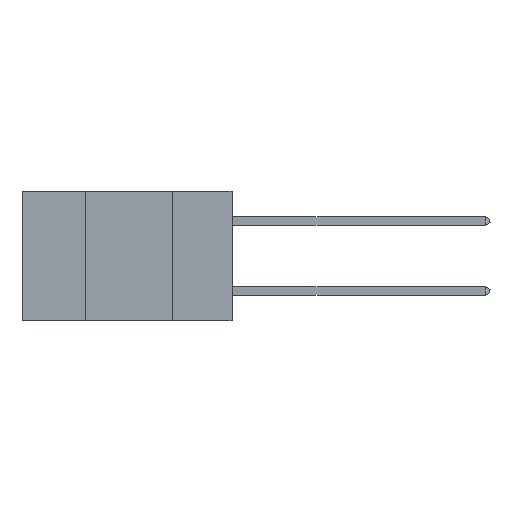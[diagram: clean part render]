
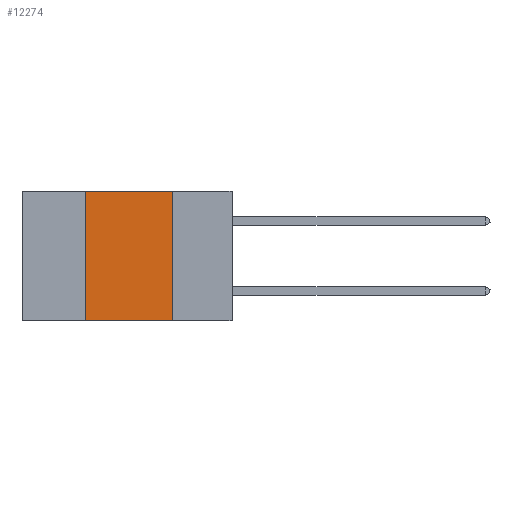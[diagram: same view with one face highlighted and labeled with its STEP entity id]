
A CAD part, left-side view. The second image highlights one B-rep face of the part: STEP entity #12274.
In plain terms, the highlighted planar face has unit normal (-1, 0, 0).
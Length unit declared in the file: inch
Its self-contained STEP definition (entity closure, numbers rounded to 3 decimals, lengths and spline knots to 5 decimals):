
#4 = EDGE_CURVE ( 'NONE', #7648, #14621, #4949, .T. ) ;
#509 = EDGE_CURVE ( 'NONE', #6425, #7648, #12445, .T. ) ;
#868 = DIRECTION ( 'NONE',  ( 0., -1., 0. ) ) ;
#1037 = EDGE_LOOP ( 'NONE', ( #7415, #4270, #7831, #11387 ) ) ;
#1238 = VECTOR ( 'NONE', #12157, 39.37008 ) ;
#1306 = FACE_OUTER_BOUND ( 'NONE', #1037, .T. ) ;
#2282 = CARTESIAN_POINT ( 'NONE',  ( 0., 0.6, 0. ) ) ;
#3212 = CARTESIAN_POINT ( 'NONE',  ( 0., 0.17, 0. ) ) ;
#3716 = LINE ( 'NONE', #16915, #10445 ) ;
#4270 = ORIENTED_EDGE ( 'NONE', *, *, #509, .F. ) ;
#4773 = CARTESIAN_POINT ( 'NONE',  ( 0., 0.42, 0. ) ) ;
#4949 = LINE ( 'NONE', #3212, #1238 ) ;
#5551 = DIRECTION ( 'NONE',  ( 0., -1., 0. ) ) ;
#5793 = PLANE ( 'NONE',  #7025 ) ;
#5878 = CARTESIAN_POINT ( 'NONE',  ( 0., 0.42, 0. ) ) ;
#6054 = LINE ( 'NONE', #5878, #16155 ) ;
#6425 = VERTEX_POINT ( 'NONE', #4773 ) ;
#7025 = AXIS2_PLACEMENT_3D ( 'NONE', #12415, #15013, #7111 ) ;
#7111 = DIRECTION ( 'NONE',  ( 0., 0., -1. ) ) ;
#7415 = ORIENTED_EDGE ( 'NONE', *, *, #4, .F. ) ;
#7648 = VERTEX_POINT ( 'NONE', #13950 ) ;
#7831 = ORIENTED_EDGE ( 'NONE', *, *, #13521, .F. ) ;
#8895 = VECTOR ( 'NONE', #5551, 39.37008 ) ;
#9934 = VERTEX_POINT ( 'NONE', #12018 ) ;
#10445 = VECTOR ( 'NONE', #868, 39.37008 ) ;
#11387 = ORIENTED_EDGE ( 'NONE', *, *, #11927, .T. ) ;
#11927 = EDGE_CURVE ( 'NONE', #9934, #14621, #3716, .T. ) ;
#12018 = CARTESIAN_POINT ( 'NONE',  ( 0., 0.42, -0.37 ) ) ;
#12157 = DIRECTION ( 'NONE',  ( 0., 0., -1. ) ) ;
#12274 = ADVANCED_FACE ( 'NONE', ( #1306 ), #5793, .F. ) ;
#12415 = CARTESIAN_POINT ( 'NONE',  ( 0., 0.6, 0. ) ) ;
#12445 = LINE ( 'NONE', #2282, #8895 ) ;
#13521 = EDGE_CURVE ( 'NONE', #9934, #6425, #6054, .T. ) ;
#13950 = CARTESIAN_POINT ( 'NONE',  ( 0., 0.17, 0. ) ) ;
#14621 = VERTEX_POINT ( 'NONE', #15917 ) ;
#15013 = DIRECTION ( 'NONE',  ( 1., 0., 0. ) ) ;
#15917 = CARTESIAN_POINT ( 'NONE',  ( 0., 0.17, -0.37 ) ) ;
#16155 = VECTOR ( 'NONE', #16418, 39.37008 ) ;
#16418 = DIRECTION ( 'NONE',  ( 0., 0., 1. ) ) ;
#16915 = CARTESIAN_POINT ( 'NONE',  ( 0., 0.6, -0.37 ) ) ;
